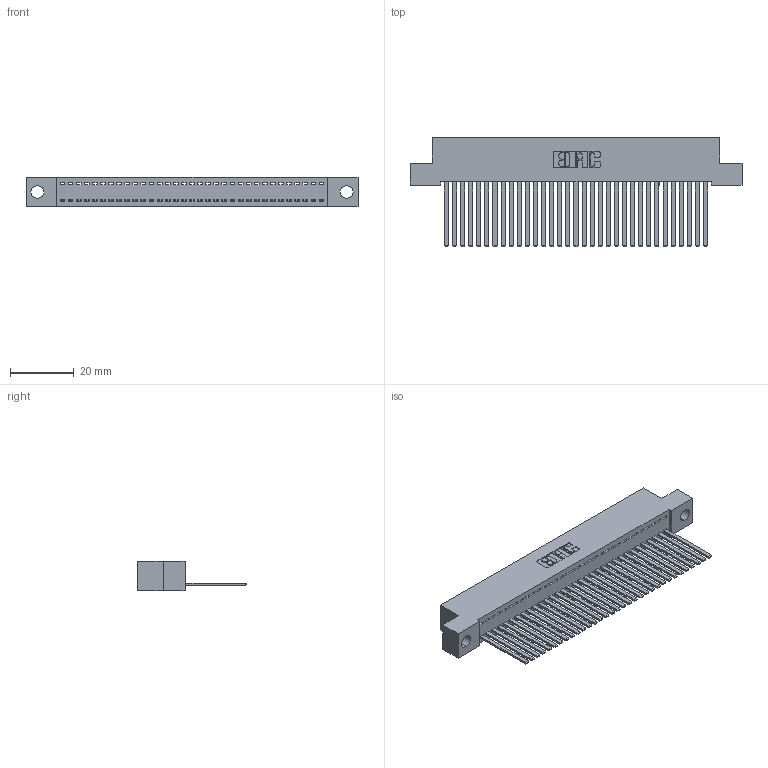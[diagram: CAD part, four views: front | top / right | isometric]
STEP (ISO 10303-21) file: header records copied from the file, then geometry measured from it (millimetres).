
FILE_DESCRIPTION (( 'STEP AP203' ), '1' );
FILE_NAME ('392-033-544-104.STEP', '2018-08-16T00:59:06', ( '' ), ( '' ), 'SwSTEP 2.0', 'SolidWorks 2016', '' );
FILE_SCHEMA (( 'CONFIG_CONTROL_DESIGN' ));
Length unit declared in the file: inch
Products named in the file (3): 342 Part_.156 TH; 345-292-001_345-293-144; 392-033-544-104
Assembly tree (34 placements, depth 2):
  392-033-544-104
    342 Part_.156 TH
    345-292-001_345-293-144  x33
Bounding box: 104.14 x 34.3 x 9.4 mm (x, y, z)
Volume: 9393 mm3; surface area: 14531.7 mm2
Topology: 34 solids, 34 shells, 1826 faces, 5513 edges, 3630 vertices
Faces by surface type: plane 1320, cylinder 506
Entity records: 21025 total; most frequent: CARTESIAN_POINT 3633, ORIENTED_EDGE 3602, DIRECTION 3079, EDGE_CURVE 1801, LINE 1677, VECTOR 1677, VERTEX_POINT 1198, AXIS2_PLACEMENT_3D 701
